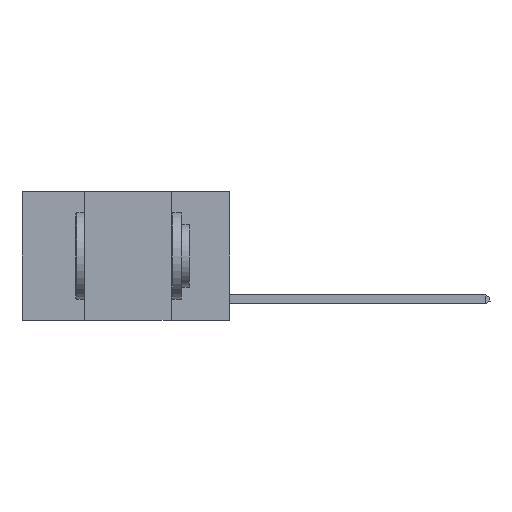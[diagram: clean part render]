
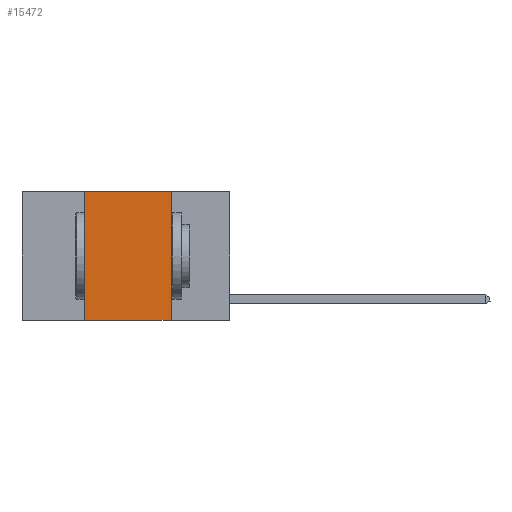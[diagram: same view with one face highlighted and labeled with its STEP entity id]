
A CAD part, left-side view. The second image highlights one B-rep face of the part: STEP entity #15472.
In plain terms, the highlighted planar face has unit normal (-1, 0, 0).
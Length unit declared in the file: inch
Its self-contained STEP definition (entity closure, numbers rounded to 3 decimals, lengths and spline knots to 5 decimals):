
#1023 = CARTESIAN_POINT ( 'NONE',  ( 0., 0.17, 0. ) ) ;
#1271 = VECTOR ( 'NONE', #16354, 39.37008 ) ;
#2312 = LINE ( 'NONE', #18432, #2677 ) ;
#2677 = VECTOR ( 'NONE', #16255, 39.37008 ) ;
#3950 = LINE ( 'NONE', #13215, #25584 ) ;
#4900 = ORIENTED_EDGE ( 'NONE', *, *, #14722, .F. ) ;
#6246 = CARTESIAN_POINT ( 'NONE',  ( 0., 0.42, -0.37 ) ) ;
#6738 = LINE ( 'NONE', #8518, #24122 ) ;
#8518 = CARTESIAN_POINT ( 'NONE',  ( 0., 0.42, 0. ) ) ;
#10153 = EDGE_CURVE ( 'NONE', #28872, #23243, #6738, .T. ) ;
#10166 = CARTESIAN_POINT ( 'NONE',  ( 0., 0.17, -0.37 ) ) ;
#13215 = CARTESIAN_POINT ( 'NONE',  ( 0., 0.17, 0. ) ) ;
#13374 = CARTESIAN_POINT ( 'NONE',  ( 0., 0.42, 0. ) ) ;
#13537 = DIRECTION ( 'NONE',  ( 0., 0., -1. ) ) ;
#13922 = CARTESIAN_POINT ( 'NONE',  ( 0., 0.6, 0. ) ) ;
#14325 = EDGE_LOOP ( 'NONE', ( #14920, #4900, #15308, #24560 ) ) ;
#14722 = EDGE_CURVE ( 'NONE', #23243, #18458, #19714, .T. ) ;
#14920 = ORIENTED_EDGE ( 'NONE', *, *, #16663, .F. ) ;
#15308 = ORIENTED_EDGE ( 'NONE', *, *, #10153, .F. ) ;
#15472 = ADVANCED_FACE ( 'NONE', ( #18596 ), #22879, .F. ) ;
#16182 = AXIS2_PLACEMENT_3D ( 'NONE', #13922, #27224, #13537 ) ;
#16255 = DIRECTION ( 'NONE',  ( 0., -1., 0. ) ) ;
#16354 = DIRECTION ( 'NONE',  ( 0., -1., 0. ) ) ;
#16663 = EDGE_CURVE ( 'NONE', #18458, #24399, #3950, .T. ) ;
#18134 = EDGE_CURVE ( 'NONE', #28872, #24399, #2312, .T. ) ;
#18432 = CARTESIAN_POINT ( 'NONE',  ( 0., 0.6, -0.37 ) ) ;
#18458 = VERTEX_POINT ( 'NONE', #1023 ) ;
#18596 = FACE_OUTER_BOUND ( 'NONE', #14325, .T. ) ;
#19714 = LINE ( 'NONE', #20614, #1271 ) ;
#20309 = DIRECTION ( 'NONE',  ( 0., 0., 1. ) ) ;
#20614 = CARTESIAN_POINT ( 'NONE',  ( 0., 0.6, 0. ) ) ;
#22879 = PLANE ( 'NONE',  #16182 ) ;
#23243 = VERTEX_POINT ( 'NONE', #13374 ) ;
#24122 = VECTOR ( 'NONE', #20309, 39.37008 ) ;
#24399 = VERTEX_POINT ( 'NONE', #10166 ) ;
#24560 = ORIENTED_EDGE ( 'NONE', *, *, #18134, .T. ) ;
#25584 = VECTOR ( 'NONE', #29067, 39.37008 ) ;
#27224 = DIRECTION ( 'NONE',  ( 1., 0., 0. ) ) ;
#28872 = VERTEX_POINT ( 'NONE', #6246 ) ;
#29067 = DIRECTION ( 'NONE',  ( 0., 0., -1. ) ) ;
